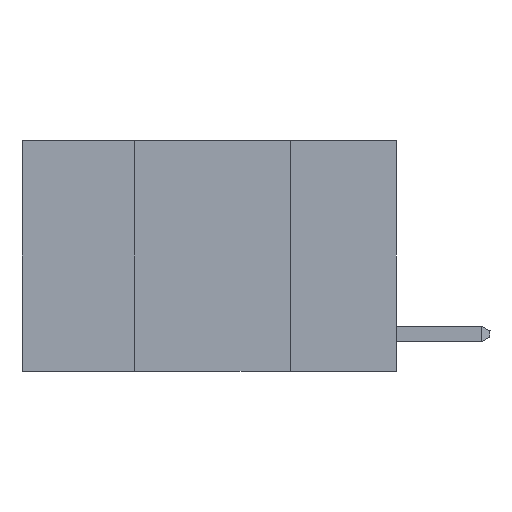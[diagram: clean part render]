
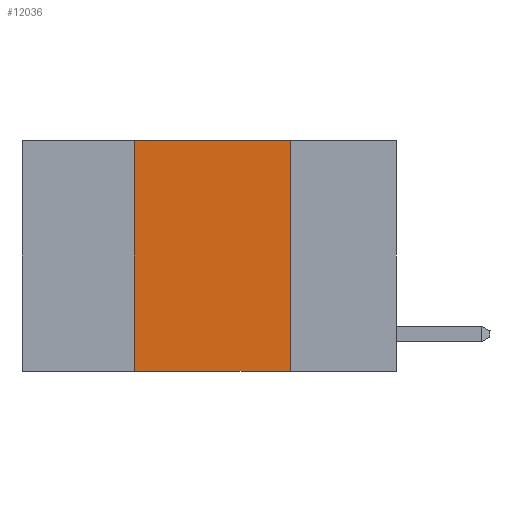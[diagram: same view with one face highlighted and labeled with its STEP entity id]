
A CAD part, left-side view. The second image highlights one B-rep face of the part: STEP entity #12036.
In plain terms, the highlighted planar face has unit normal (-1, 0, 0).
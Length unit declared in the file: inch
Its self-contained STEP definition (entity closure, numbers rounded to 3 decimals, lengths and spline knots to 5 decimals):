
#743 = ORIENTED_EDGE ( 'NONE', *, *, #10733, .F. ) ;
#764 = DIRECTION ( 'NONE',  ( 1., 0., 0. ) ) ;
#1019 = VERTEX_POINT ( 'NONE', #9944 ) ;
#1384 = CARTESIAN_POINT ( 'NONE',  ( 0., 0.42, 0. ) ) ;
#1452 = CARTESIAN_POINT ( 'NONE',  ( 0., 0.6, 0. ) ) ;
#2132 = CARTESIAN_POINT ( 'NONE',  ( 0., 0.17, 0. ) ) ;
#2135 = LINE ( 'NONE', #5620, #9555 ) ;
#2673 = ORIENTED_EDGE ( 'NONE', *, *, #10671, .F. ) ;
#3364 = CARTESIAN_POINT ( 'NONE',  ( 0., 0.42, 0. ) ) ;
#4232 = VECTOR ( 'NONE', #14335, 39.37008 ) ;
#4361 = VERTEX_POINT ( 'NONE', #12793 ) ;
#4871 = LINE ( 'NONE', #1384, #12958 ) ;
#5168 = PLANE ( 'NONE',  #14137 ) ;
#5417 = VECTOR ( 'NONE', #7039, 39.37008 ) ;
#5486 = DIRECTION ( 'NONE',  ( 0., 0., -1. ) ) ;
#5620 = CARTESIAN_POINT ( 'NONE',  ( 0., 0.6, -0.37 ) ) ;
#6202 = VERTEX_POINT ( 'NONE', #3364 ) ;
#6332 = ORIENTED_EDGE ( 'NONE', *, *, #7454, .F. ) ;
#7039 = DIRECTION ( 'NONE',  ( 0., 0., -1. ) ) ;
#7072 = VERTEX_POINT ( 'NONE', #8057 ) ;
#7454 = EDGE_CURVE ( 'NONE', #1019, #7072, #10242, .T. ) ;
#8057 = CARTESIAN_POINT ( 'NONE',  ( 0., 0.17, -0.37 ) ) ;
#8330 = EDGE_LOOP ( 'NONE', ( #6332, #743, #2673, #9410 ) ) ;
#8784 = EDGE_CURVE ( 'NONE', #4361, #7072, #2135, .T. ) ;
#8902 = CARTESIAN_POINT ( 'NONE',  ( 0., 0.6, 0. ) ) ;
#9410 = ORIENTED_EDGE ( 'NONE', *, *, #8784, .T. ) ;
#9555 = VECTOR ( 'NONE', #10245, 39.37008 ) ;
#9726 = LINE ( 'NONE', #1452, #4232 ) ;
#9944 = CARTESIAN_POINT ( 'NONE',  ( 0., 0.17, 0. ) ) ;
#10242 = LINE ( 'NONE', #2132, #5417 ) ;
#10245 = DIRECTION ( 'NONE',  ( 0., -1., 0. ) ) ;
#10646 = DIRECTION ( 'NONE',  ( 0., 0., 1. ) ) ;
#10671 = EDGE_CURVE ( 'NONE', #4361, #6202, #4871, .T. ) ;
#10733 = EDGE_CURVE ( 'NONE', #6202, #1019, #9726, .T. ) ;
#12036 = ADVANCED_FACE ( 'NONE', ( #14730 ), #5168, .F. ) ;
#12793 = CARTESIAN_POINT ( 'NONE',  ( 0., 0.42, -0.37 ) ) ;
#12958 = VECTOR ( 'NONE', #10646, 39.37008 ) ;
#14137 = AXIS2_PLACEMENT_3D ( 'NONE', #8902, #764, #5486 ) ;
#14335 = DIRECTION ( 'NONE',  ( 0., -1., 0. ) ) ;
#14730 = FACE_OUTER_BOUND ( 'NONE', #8330, .T. ) ;
